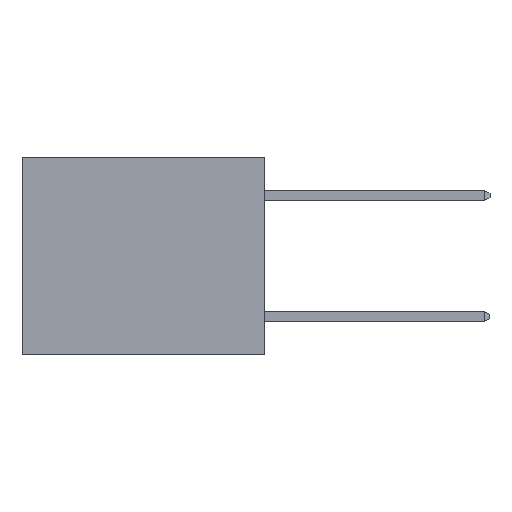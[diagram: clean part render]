
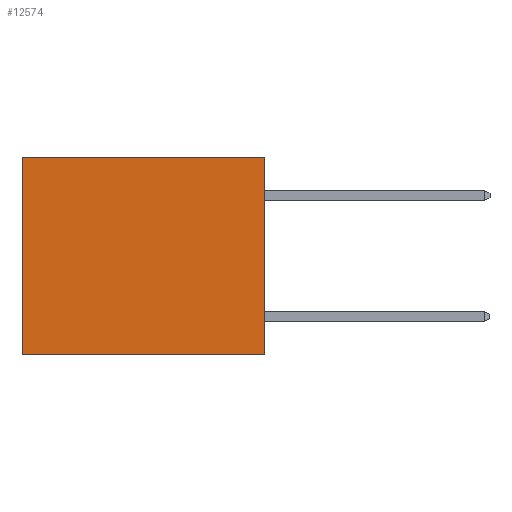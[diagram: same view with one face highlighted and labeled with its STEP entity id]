
A CAD part, left-side view. The second image highlights one B-rep face of the part: STEP entity #12574.
In plain terms, the highlighted planar face has unit normal (-1, 0, 0).
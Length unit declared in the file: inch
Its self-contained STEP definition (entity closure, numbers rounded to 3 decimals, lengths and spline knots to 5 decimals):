
#732 = LINE ( 'NONE', #10600, #8033 ) ;
#889 = ORIENTED_EDGE ( 'NONE', *, *, #1903, .T. ) ;
#956 = AXIS2_PLACEMENT_3D ( 'NONE', #2667, #12029, #1645 ) ;
#1515 = DIRECTION ( 'NONE',  ( 0., 0., -1. ) ) ;
#1645 = DIRECTION ( 'NONE',  ( 0., 0., -1. ) ) ;
#1878 = VERTEX_POINT ( 'NONE', #10525 ) ;
#1903 = EDGE_CURVE ( 'NONE', #4515, #13429, #7212, .T. ) ;
#2525 = DIRECTION ( 'NONE',  ( 0., 0., -1. ) ) ;
#2667 = CARTESIAN_POINT ( 'NONE',  ( 0.3165, 0., -0.49 ) ) ;
#2854 = DIRECTION ( 'NONE',  ( 0., 1., 0. ) ) ;
#2995 = ORIENTED_EDGE ( 'NONE', *, *, #12863, .F. ) ;
#4515 = VERTEX_POINT ( 'NONE', #5901 ) ;
#5404 = CARTESIAN_POINT ( 'NONE',  ( 0.3165, 0.6, -0.49 ) ) ;
#5901 = CARTESIAN_POINT ( 'NONE',  ( 0.3165, 0.6, 0. ) ) ;
#5907 = VECTOR ( 'NONE', #7946, 39.37008 ) ;
#6771 = ORIENTED_EDGE ( 'NONE', *, *, #7482, .F. ) ;
#7190 = CARTESIAN_POINT ( 'NONE',  ( 0.3165, 0.6, -0.49 ) ) ;
#7212 = LINE ( 'NONE', #7190, #14233 ) ;
#7482 = EDGE_CURVE ( 'NONE', #1878, #13429, #11465, .T. ) ;
#7487 = EDGE_LOOP ( 'NONE', ( #889, #6771, #2995, #13296 ) ) ;
#7946 = DIRECTION ( 'NONE',  ( 0., 1., 0. ) ) ;
#7981 = CARTESIAN_POINT ( 'NONE',  ( 0.3165, 0., 0. ) ) ;
#8033 = VECTOR ( 'NONE', #2525, 39.37008 ) ;
#8052 = FACE_OUTER_BOUND ( 'NONE', #7487, .T. ) ;
#8898 = CARTESIAN_POINT ( 'NONE',  ( 0.3165, 0., 0. ) ) ;
#8982 = LINE ( 'NONE', #8898, #5907 ) ;
#9484 = VECTOR ( 'NONE', #2854, 39.37008 ) ;
#10525 = CARTESIAN_POINT ( 'NONE',  ( 0.3165, 0., -0.49 ) ) ;
#10600 = CARTESIAN_POINT ( 'NONE',  ( 0.3165, 0., -0.49 ) ) ;
#10733 = EDGE_CURVE ( 'NONE', #13053, #4515, #8982, .T. ) ;
#11465 = LINE ( 'NONE', #14253, #9484 ) ;
#12029 = DIRECTION ( 'NONE',  ( 1., 0., 0. ) ) ;
#12574 = ADVANCED_FACE ( 'NONE', ( #8052 ), #14165, .F. ) ;
#12863 = EDGE_CURVE ( 'NONE', #13053, #1878, #732, .T. ) ;
#13053 = VERTEX_POINT ( 'NONE', #7981 ) ;
#13296 = ORIENTED_EDGE ( 'NONE', *, *, #10733, .T. ) ;
#13429 = VERTEX_POINT ( 'NONE', #5404 ) ;
#14165 = PLANE ( 'NONE',  #956 ) ;
#14233 = VECTOR ( 'NONE', #1515, 39.37008 ) ;
#14253 = CARTESIAN_POINT ( 'NONE',  ( 0.3165, 0., -0.49 ) ) ;
